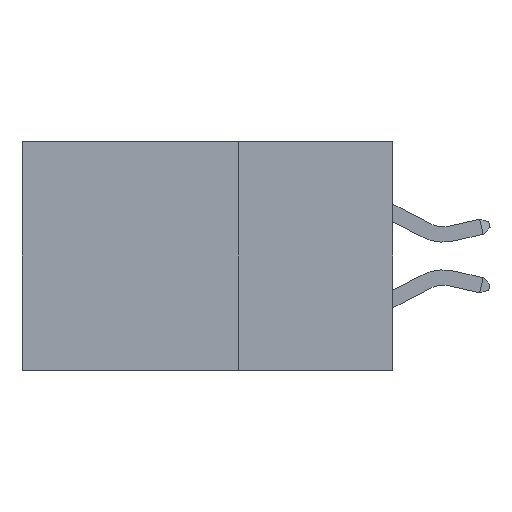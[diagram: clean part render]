
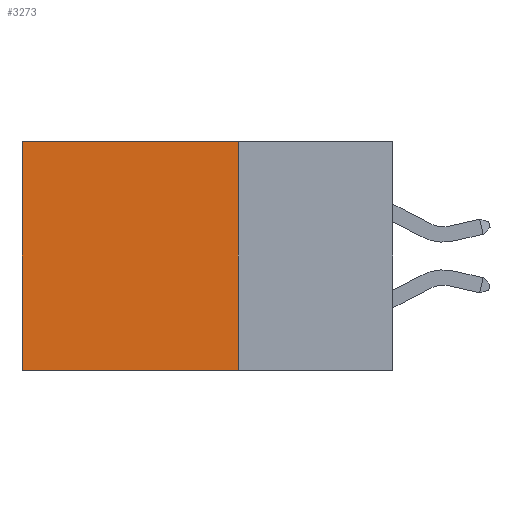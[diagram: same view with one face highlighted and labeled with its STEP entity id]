
A CAD part, left-side view. The second image highlights one B-rep face of the part: STEP entity #3273.
In plain terms, the highlighted planar face has unit normal (-1, 0, 0).
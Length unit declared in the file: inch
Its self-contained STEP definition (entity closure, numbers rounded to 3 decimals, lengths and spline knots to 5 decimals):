
#388 = ORIENTED_EDGE ( 'NONE', *, *, #5818, .F. ) ;
#446 = ORIENTED_EDGE ( 'NONE', *, *, #12502, .T. ) ;
#2203 = VERTEX_POINT ( 'NONE', #18309 ) ;
#2277 = DIRECTION ( 'NONE',  ( 0., 0., -1. ) ) ;
#2496 = EDGE_CURVE ( 'NONE', #14618, #2203, #13605, .T. ) ;
#2546 = EDGE_LOOP ( 'NONE', ( #6379, #388, #14487, #446 ) ) ;
#3273 = ADVANCED_FACE ( 'NONE', ( #18705 ), #15879, .F. ) ;
#3444 = VECTOR ( 'NONE', #4916, 39.37008 ) ;
#4916 = DIRECTION ( 'NONE',  ( 0., 1., 0. ) ) ;
#5200 = DIRECTION ( 'NONE',  ( 1., 0., 0. ) ) ;
#5818 = EDGE_CURVE ( 'NONE', #2203, #10680, #6469, .T. ) ;
#5830 = LINE ( 'NONE', #9658, #14190 ) ;
#6142 = CARTESIAN_POINT ( 'NONE',  ( 0.2875, 0.25, 0. ) ) ;
#6379 = ORIENTED_EDGE ( 'NONE', *, *, #9141, .T. ) ;
#6469 = LINE ( 'NONE', #17053, #3444 ) ;
#8186 = AXIS2_PLACEMENT_3D ( 'NONE', #12837, #5200, #2277 ) ;
#9141 = EDGE_CURVE ( 'NONE', #12882, #10680, #10683, .T. ) ;
#9658 = CARTESIAN_POINT ( 'NONE',  ( 0.2875, 0.25, 0. ) ) ;
#10680 = VERTEX_POINT ( 'NONE', #14536 ) ;
#10683 = LINE ( 'NONE', #12440, #18513 ) ;
#12121 = DIRECTION ( 'NONE',  ( 0., 0., -1. ) ) ;
#12343 = DIRECTION ( 'NONE',  ( 0., 0., -1. ) ) ;
#12440 = CARTESIAN_POINT ( 'NONE',  ( 0.2875, 0.6, 0. ) ) ;
#12502 = EDGE_CURVE ( 'NONE', #14618, #12882, #5830, .T. ) ;
#12837 = CARTESIAN_POINT ( 'NONE',  ( 0.2875, 0.25, 0. ) ) ;
#12882 = VERTEX_POINT ( 'NONE', #13156 ) ;
#12912 = DIRECTION ( 'NONE',  ( 0., 1., 0. ) ) ;
#12944 = CARTESIAN_POINT ( 'NONE',  ( 0.2875, 0.25, 0. ) ) ;
#13156 = CARTESIAN_POINT ( 'NONE',  ( 0.2875, 0.6, 0. ) ) ;
#13605 = LINE ( 'NONE', #6142, #14195 ) ;
#14190 = VECTOR ( 'NONE', #12912, 39.37008 ) ;
#14195 = VECTOR ( 'NONE', #12121, 39.37008 ) ;
#14487 = ORIENTED_EDGE ( 'NONE', *, *, #2496, .F. ) ;
#14536 = CARTESIAN_POINT ( 'NONE',  ( 0.2875, 0.6, -0.37 ) ) ;
#14618 = VERTEX_POINT ( 'NONE', #12944 ) ;
#15879 = PLANE ( 'NONE',  #8186 ) ;
#17053 = CARTESIAN_POINT ( 'NONE',  ( 0.2875, 0.25, -0.37 ) ) ;
#18309 = CARTESIAN_POINT ( 'NONE',  ( 0.2875, 0.25, -0.37 ) ) ;
#18513 = VECTOR ( 'NONE', #12343, 39.37008 ) ;
#18705 = FACE_OUTER_BOUND ( 'NONE', #2546, .T. ) ;
